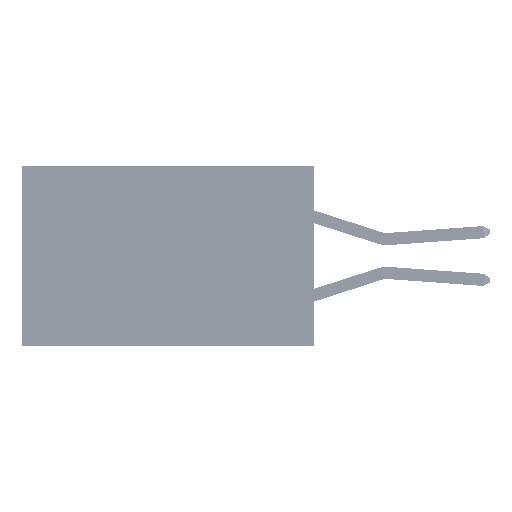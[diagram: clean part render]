
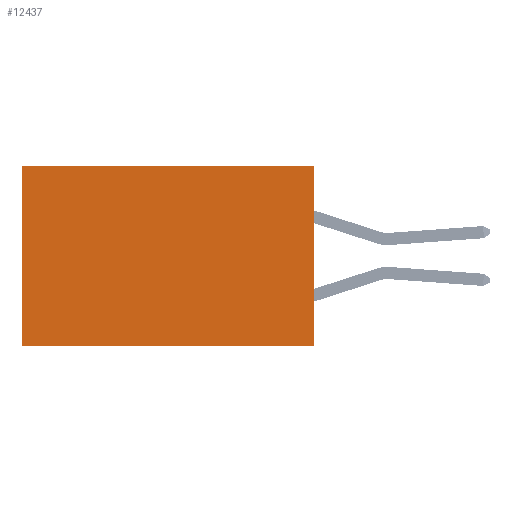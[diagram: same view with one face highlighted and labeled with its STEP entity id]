
A CAD part, left-side view. The second image highlights one B-rep face of the part: STEP entity #12437.
In plain terms, the highlighted planar face has unit normal (-1, 0, 0).
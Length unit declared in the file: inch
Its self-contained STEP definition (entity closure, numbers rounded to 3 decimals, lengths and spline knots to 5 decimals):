
#1134 = CARTESIAN_POINT ( 'NONE',  ( 0.2875, 0., 0. ) ) ;
#2129 = LINE ( 'NONE', #27701, #45340 ) ;
#2327 = CARTESIAN_POINT ( 'NONE',  ( 0.2875, 0.6, 0. ) ) ;
#3912 = EDGE_CURVE ( 'NONE', #41830, #40935, #20460, .T. ) ;
#3973 = LINE ( 'NONE', #1134, #46499 ) ;
#5043 = CARTESIAN_POINT ( 'NONE',  ( 0.2875, 0., 0. ) ) ;
#5230 = CARTESIAN_POINT ( 'NONE',  ( 0.2875, 0., 0. ) ) ;
#10159 = VECTOR ( 'NONE', #21349, 39.37008 ) ;
#12437 = ADVANCED_FACE ( 'NONE', ( #41185 ), #48294, .F. ) ;
#13851 = VERTEX_POINT ( 'NONE', #2327 ) ;
#14613 = ORIENTED_EDGE ( 'NONE', *, *, #28976, .F. ) ;
#17300 = DIRECTION ( 'NONE',  ( 1., 0., 0. ) ) ;
#17563 = EDGE_CURVE ( 'NONE', #34562, #13851, #29262, .T. ) ;
#18808 = AXIS2_PLACEMENT_3D ( 'NONE', #44255, #17300, #44594 ) ;
#20460 = LINE ( 'NONE', #36720, #10159 ) ;
#20759 = DIRECTION ( 'NONE',  ( 0., 0., -1. ) ) ;
#20790 = ORIENTED_EDGE ( 'NONE', *, *, #3912, .F. ) ;
#21349 = DIRECTION ( 'NONE',  ( 0., 1., 0. ) ) ;
#22876 = CARTESIAN_POINT ( 'NONE',  ( 0.2875, 0., -0.37 ) ) ;
#27701 = CARTESIAN_POINT ( 'NONE',  ( 0.2875, 0.6, 0. ) ) ;
#28976 = EDGE_CURVE ( 'NONE', #34562, #41830, #3973, .T. ) ;
#29262 = LINE ( 'NONE', #5230, #31052 ) ;
#29792 = ORIENTED_EDGE ( 'NONE', *, *, #17563, .T. ) ;
#31052 = VECTOR ( 'NONE', #40200, 39.37008 ) ;
#34562 = VERTEX_POINT ( 'NONE', #5043 ) ;
#35966 = DIRECTION ( 'NONE',  ( 0., 0., -1. ) ) ;
#36594 = EDGE_CURVE ( 'NONE', #13851, #40935, #2129, .T. ) ;
#36720 = CARTESIAN_POINT ( 'NONE',  ( 0.2875, 0., -0.37 ) ) ;
#38734 = ORIENTED_EDGE ( 'NONE', *, *, #36594, .T. ) ;
#40200 = DIRECTION ( 'NONE',  ( 0., 1., 0. ) ) ;
#40935 = VERTEX_POINT ( 'NONE', #48454 ) ;
#41185 = FACE_OUTER_BOUND ( 'NONE', #48037, .T. ) ;
#41830 = VERTEX_POINT ( 'NONE', #22876 ) ;
#44255 = CARTESIAN_POINT ( 'NONE',  ( 0.2875, 0., 0. ) ) ;
#44594 = DIRECTION ( 'NONE',  ( 0., 0., -1. ) ) ;
#45340 = VECTOR ( 'NONE', #35966, 39.37008 ) ;
#46499 = VECTOR ( 'NONE', #20759, 39.37008 ) ;
#48037 = EDGE_LOOP ( 'NONE', ( #38734, #20790, #14613, #29792 ) ) ;
#48294 = PLANE ( 'NONE',  #18808 ) ;
#48454 = CARTESIAN_POINT ( 'NONE',  ( 0.2875, 0.6, -0.37 ) ) ;
